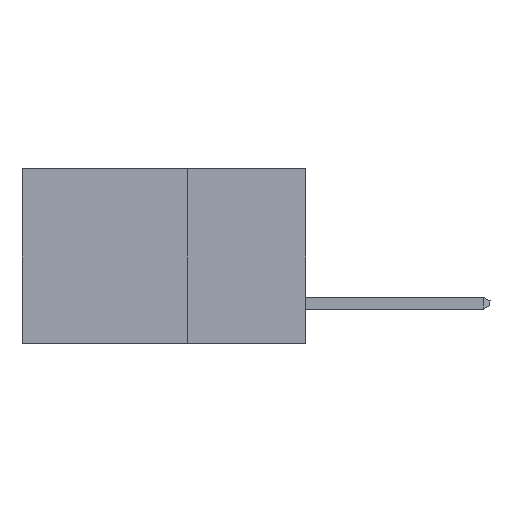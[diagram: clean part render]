
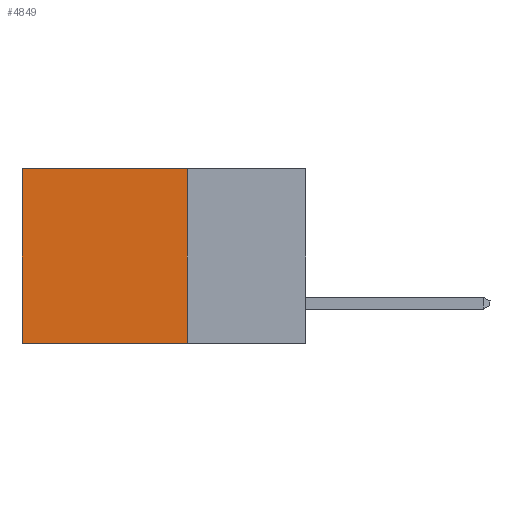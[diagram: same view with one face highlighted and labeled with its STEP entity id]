
A CAD part, left-side view. The second image highlights one B-rep face of the part: STEP entity #4849.
In plain terms, the highlighted planar face has unit normal (-1, 0, 0).
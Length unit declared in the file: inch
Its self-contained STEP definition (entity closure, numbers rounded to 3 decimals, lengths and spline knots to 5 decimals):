
#113 = LINE ( 'NONE', #18236, #18074 ) ;
#943 = CARTESIAN_POINT ( 'NONE',  ( 0.2615, 0.25, -0.37 ) ) ;
#990 = VERTEX_POINT ( 'NONE', #6004 ) ;
#3300 = EDGE_CURVE ( 'NONE', #16067, #990, #7006, .T. ) ;
#3451 = DIRECTION ( 'NONE',  ( 1., 0., 0. ) ) ;
#3659 = FACE_OUTER_BOUND ( 'NONE', #18614, .T. ) ;
#3680 = VECTOR ( 'NONE', #18908, 39.37008 ) ;
#4110 = ORIENTED_EDGE ( 'NONE', *, *, #12950, .F. ) ;
#4374 = VECTOR ( 'NONE', #19451, 39.37008 ) ;
#4630 = LINE ( 'NONE', #18057, #6782 ) ;
#4849 = ADVANCED_FACE ( 'NONE', ( #3659 ), #6524, .F. ) ;
#5500 = CARTESIAN_POINT ( 'NONE',  ( 0.2615, 0.6, 0. ) ) ;
#6004 = CARTESIAN_POINT ( 'NONE',  ( 0.2615, 0.25, -0.37 ) ) ;
#6208 = DIRECTION ( 'NONE',  ( 0., 0., -1. ) ) ;
#6524 = PLANE ( 'NONE',  #10523 ) ;
#6712 = VERTEX_POINT ( 'NONE', #5500 ) ;
#6782 = VECTOR ( 'NONE', #6208, 39.37008 ) ;
#7006 = LINE ( 'NONE', #943, #4374 ) ;
#8241 = LINE ( 'NONE', #9939, #3680 ) ;
#8965 = CARTESIAN_POINT ( 'NONE',  ( 0.2615, 0.25, 0. ) ) ;
#9939 = CARTESIAN_POINT ( 'NONE',  ( 0.2615, 0.25, -0.37 ) ) ;
#10523 = AXIS2_PLACEMENT_3D ( 'NONE', #16873, #3451, #11195 ) ;
#10777 = EDGE_CURVE ( 'NONE', #6712, #12922, #4630, .T. ) ;
#11195 = DIRECTION ( 'NONE',  ( 0., 0., -1. ) ) ;
#11484 = ORIENTED_EDGE ( 'NONE', *, *, #10777, .T. ) ;
#12922 = VERTEX_POINT ( 'NONE', #15613 ) ;
#12950 = EDGE_CURVE ( 'NONE', #990, #12922, #8241, .T. ) ;
#12964 = ORIENTED_EDGE ( 'NONE', *, *, #18625, .T. ) ;
#13669 = ORIENTED_EDGE ( 'NONE', *, *, #3300, .F. ) ;
#13751 = DIRECTION ( 'NONE',  ( 0., 1., 0. ) ) ;
#15613 = CARTESIAN_POINT ( 'NONE',  ( 0.2615, 0.6, -0.37 ) ) ;
#16067 = VERTEX_POINT ( 'NONE', #8965 ) ;
#16873 = CARTESIAN_POINT ( 'NONE',  ( 0.2615, 0.25, -0.37 ) ) ;
#18057 = CARTESIAN_POINT ( 'NONE',  ( 0.2615, 0.6, -0.37 ) ) ;
#18074 = VECTOR ( 'NONE', #13751, 39.37008 ) ;
#18236 = CARTESIAN_POINT ( 'NONE',  ( 0.2615, 0.25, 0. ) ) ;
#18614 = EDGE_LOOP ( 'NONE', ( #11484, #4110, #13669, #12964 ) ) ;
#18625 = EDGE_CURVE ( 'NONE', #16067, #6712, #113, .T. ) ;
#18908 = DIRECTION ( 'NONE',  ( 0., 1., 0. ) ) ;
#19451 = DIRECTION ( 'NONE',  ( 0., 0., -1. ) ) ;
